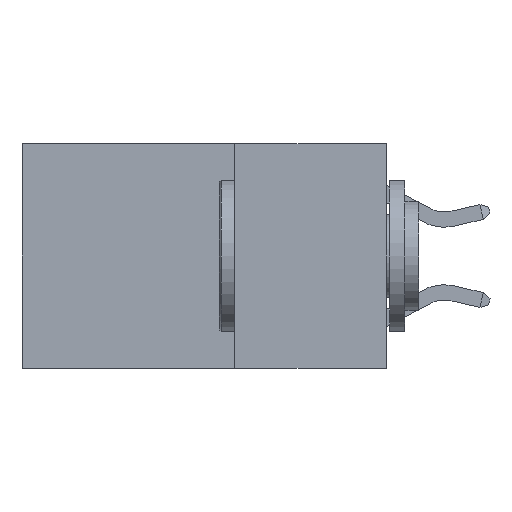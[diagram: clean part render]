
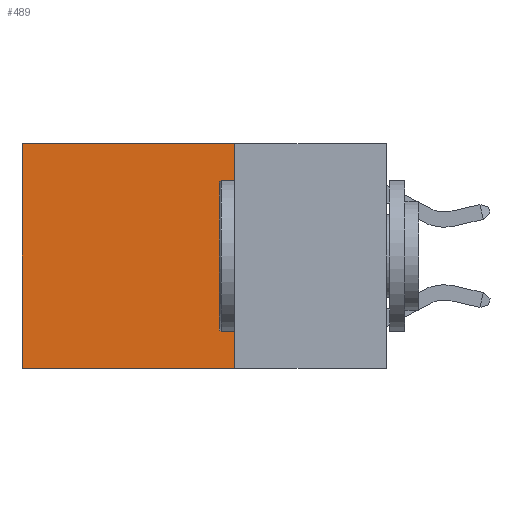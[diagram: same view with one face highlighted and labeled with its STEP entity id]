
A CAD part, left-side view. The second image highlights one B-rep face of the part: STEP entity #489.
In plain terms, the highlighted planar face has unit normal (-1, 0, 0).
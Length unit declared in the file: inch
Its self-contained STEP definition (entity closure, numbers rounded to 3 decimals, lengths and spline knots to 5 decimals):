
#382 = DIRECTION ( 'NONE',  ( 0., 1., 0. ) ) ;
#489 = ADVANCED_FACE ( 'NONE', ( #8856 ), #6359, .F. ) ;
#676 = EDGE_CURVE ( 'NONE', #9079, #5001, #11703, .T. ) ;
#926 = EDGE_CURVE ( 'NONE', #5001, #10775, #9813, .T. ) ;
#1012 = VECTOR ( 'NONE', #382, 39.37008 ) ;
#1262 = CARTESIAN_POINT ( 'NONE',  ( 0.2625, 0.25, -0.37 ) ) ;
#1591 = VECTOR ( 'NONE', #11457, 39.37008 ) ;
#1863 = CARTESIAN_POINT ( 'NONE',  ( 0.2625, 0.6, 0. ) ) ;
#1886 = LINE ( 'NONE', #10612, #1591 ) ;
#2269 = CARTESIAN_POINT ( 'NONE',  ( 0.2625, 0.6, -0.37 ) ) ;
#2490 = CARTESIAN_POINT ( 'NONE',  ( 0.2625, 0.25, 0. ) ) ;
#2494 = DIRECTION ( 'NONE',  ( 1., 0., 0. ) ) ;
#2994 = EDGE_CURVE ( 'NONE', #5439, #10775, #1886, .T. ) ;
#4005 = ORIENTED_EDGE ( 'NONE', *, *, #2994, .T. ) ;
#4022 = CARTESIAN_POINT ( 'NONE',  ( 0.2625, 0.25, -0.37 ) ) ;
#4192 = DIRECTION ( 'NONE',  ( 0., 1., 0. ) ) ;
#5001 = VERTEX_POINT ( 'NONE', #4022 ) ;
#5439 = VERTEX_POINT ( 'NONE', #1863 ) ;
#5859 = CARTESIAN_POINT ( 'NONE',  ( 0.2625, 0.25, 0. ) ) ;
#5888 = ORIENTED_EDGE ( 'NONE', *, *, #926, .F. ) ;
#6359 = PLANE ( 'NONE',  #7955 ) ;
#6611 = DIRECTION ( 'NONE',  ( 0., 0., -1. ) ) ;
#7039 = CARTESIAN_POINT ( 'NONE',  ( 0.2625, 0.25, 0. ) ) ;
#7146 = CARTESIAN_POINT ( 'NONE',  ( 0.2625, 0.25, 0. ) ) ;
#7557 = EDGE_LOOP ( 'NONE', ( #4005, #5888, #7635, #10845 ) ) ;
#7635 = ORIENTED_EDGE ( 'NONE', *, *, #676, .F. ) ;
#7955 = AXIS2_PLACEMENT_3D ( 'NONE', #7146, #2494, #8266 ) ;
#8266 = DIRECTION ( 'NONE',  ( 0., 0., -1. ) ) ;
#8719 = EDGE_CURVE ( 'NONE', #9079, #5439, #10620, .T. ) ;
#8856 = FACE_OUTER_BOUND ( 'NONE', #7557, .T. ) ;
#9079 = VERTEX_POINT ( 'NONE', #5859 ) ;
#9813 = LINE ( 'NONE', #1262, #11561 ) ;
#10612 = CARTESIAN_POINT ( 'NONE',  ( 0.2625, 0.6, 0. ) ) ;
#10620 = LINE ( 'NONE', #7039, #1012 ) ;
#10775 = VERTEX_POINT ( 'NONE', #2269 ) ;
#10845 = ORIENTED_EDGE ( 'NONE', *, *, #8719, .T. ) ;
#11435 = VECTOR ( 'NONE', #6611, 39.37008 ) ;
#11457 = DIRECTION ( 'NONE',  ( 0., 0., -1. ) ) ;
#11561 = VECTOR ( 'NONE', #4192, 39.37008 ) ;
#11703 = LINE ( 'NONE', #2490, #11435 ) ;
